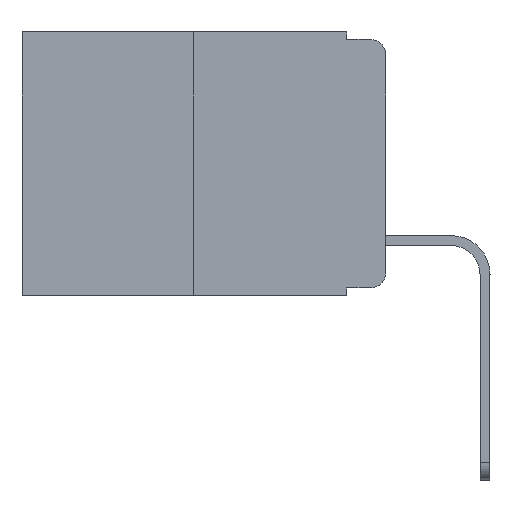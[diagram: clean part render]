
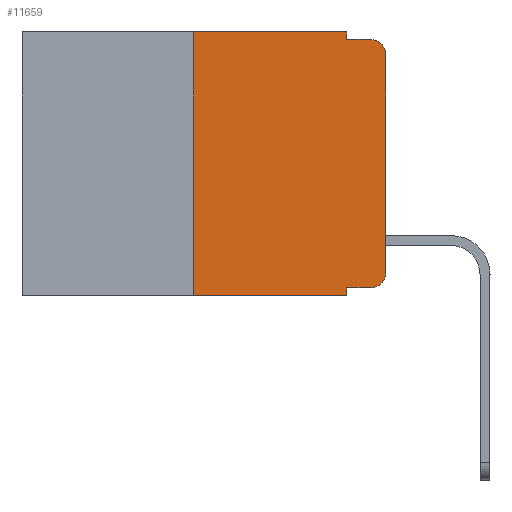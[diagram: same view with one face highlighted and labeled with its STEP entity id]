
A CAD part, left-side view. The second image highlights one B-rep face of the part: STEP entity #11659.
In plain terms, the highlighted planar face has unit normal (-1, 0, 0).
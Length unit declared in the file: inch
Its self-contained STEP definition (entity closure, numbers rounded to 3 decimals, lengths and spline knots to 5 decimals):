
#496 = DIRECTION ( 'NONE',  ( 1., 0., 0. ) ) ;
#709 = EDGE_LOOP ( 'NONE', ( #11144, #2116, #13449, #13961, #7534, #15008, #7653, #3943, #11089, #6713 ) ) ;
#839 = EDGE_CURVE ( 'NONE', #9653, #6945, #1702, .T. ) ;
#901 = EDGE_CURVE ( 'NONE', #14764, #1502, #4302, .T. ) ;
#1094 = CARTESIAN_POINT ( 'NONE',  ( 0., 0., 0. ) ) ;
#1298 = CARTESIAN_POINT ( 'NONE',  ( 0., 0.02, -0.333 ) ) ;
#1502 = VERTEX_POINT ( 'NONE', #8066 ) ;
#1522 = CARTESIAN_POINT ( 'NONE',  ( 0., 0.051, -0.01 ) ) ;
#1702 = CIRCLE ( 'NONE', #11332, 0.02 ) ;
#1748 = CARTESIAN_POINT ( 'NONE',  ( 0., 0.25, -0.343 ) ) ;
#1807 = CIRCLE ( 'NONE', #9581, 0.02 ) ;
#2116 = ORIENTED_EDGE ( 'NONE', *, *, #839, .T. ) ;
#2292 = VECTOR ( 'NONE', #12016, 39.37008 ) ;
#2937 = VERTEX_POINT ( 'NONE', #1298 ) ;
#3017 = DIRECTION ( 'NONE',  ( 0., -1., 0. ) ) ;
#3108 = CARTESIAN_POINT ( 'NONE',  ( 0., 0.473, 0. ) ) ;
#3184 = LINE ( 'NONE', #3108, #8839 ) ;
#3336 = DIRECTION ( 'NONE',  ( 0., 0., -1. ) ) ;
#3429 = CARTESIAN_POINT ( 'NONE',  ( 0., 0.051, 0. ) ) ;
#3559 = EDGE_CURVE ( 'NONE', #8387, #2937, #8196, .T. ) ;
#3943 = ORIENTED_EDGE ( 'NONE', *, *, #6161, .F. ) ;
#3948 = CARTESIAN_POINT ( 'NONE',  ( 0., 0.25, 0. ) ) ;
#4044 = CARTESIAN_POINT ( 'NONE',  ( 0., 0.051, -0.333 ) ) ;
#4079 = PLANE ( 'NONE',  #4419 ) ;
#4130 = DIRECTION ( 'NONE',  ( 0., 0., -1. ) ) ;
#4302 = LINE ( 'NONE', #6853, #14063 ) ;
#4419 = AXIS2_PLACEMENT_3D ( 'NONE', #7736, #496, #4130 ) ;
#4475 = DIRECTION ( 'NONE',  ( 0., -1., 0. ) ) ;
#4555 = CARTESIAN_POINT ( 'NONE',  ( 0., 0.25, 0. ) ) ;
#5433 = LINE ( 'NONE', #8692, #8498 ) ;
#5662 = LINE ( 'NONE', #1522, #7557 ) ;
#5698 = EDGE_CURVE ( 'NONE', #9456, #6945, #5662, .T. ) ;
#5762 = EDGE_CURVE ( 'NONE', #14777, #9653, #15029, .T. ) ;
#6000 = CARTESIAN_POINT ( 'NONE',  ( 0., 0.051, 0. ) ) ;
#6161 = EDGE_CURVE ( 'NONE', #8387, #1502, #9674, .T. ) ;
#6273 = FACE_OUTER_BOUND ( 'NONE', #709, .T. ) ;
#6713 = ORIENTED_EDGE ( 'NONE', *, *, #11077, .T. ) ;
#6776 = CARTESIAN_POINT ( 'NONE',  ( 0., 0.02, -0.313 ) ) ;
#6831 = CARTESIAN_POINT ( 'NONE',  ( 0., 0.051, -0.333 ) ) ;
#6853 = CARTESIAN_POINT ( 'NONE',  ( 0., 0.473, -0.343 ) ) ;
#6945 = VERTEX_POINT ( 'NONE', #12010 ) ;
#7286 = DIRECTION ( 'NONE',  ( 0., 0., -1. ) ) ;
#7534 = ORIENTED_EDGE ( 'NONE', *, *, #8431, .F. ) ;
#7557 = VECTOR ( 'NONE', #8630, 39.37008 ) ;
#7653 = ORIENTED_EDGE ( 'NONE', *, *, #901, .T. ) ;
#7736 = CARTESIAN_POINT ( 'NONE',  ( 0., 0.473, 0. ) ) ;
#8062 = VECTOR ( 'NONE', #9915, 39.37008 ) ;
#8066 = CARTESIAN_POINT ( 'NONE',  ( 0., 0.051, -0.343 ) ) ;
#8078 = CARTESIAN_POINT ( 'NONE',  ( 0., 0., -0.03 ) ) ;
#8196 = LINE ( 'NONE', #6831, #8738 ) ;
#8387 = VERTEX_POINT ( 'NONE', #4044 ) ;
#8431 = EDGE_CURVE ( 'NONE', #10648, #10008, #3184, .T. ) ;
#8498 = VECTOR ( 'NONE', #11091, 39.37008 ) ;
#8630 = DIRECTION ( 'NONE',  ( 0., -1., 0. ) ) ;
#8692 = CARTESIAN_POINT ( 'NONE',  ( 0., 0.051, 0. ) ) ;
#8738 = VECTOR ( 'NONE', #10573, 39.37008 ) ;
#8839 = VECTOR ( 'NONE', #3017, 39.37008 ) ;
#9292 = CARTESIAN_POINT ( 'NONE',  ( 0., 0.02, -0.03 ) ) ;
#9434 = DIRECTION ( 'NONE',  ( -1., 0., 0. ) ) ;
#9456 = VERTEX_POINT ( 'NONE', #10021 ) ;
#9581 = AXIS2_PLACEMENT_3D ( 'NONE', #6776, #12762, #10415 ) ;
#9653 = VERTEX_POINT ( 'NONE', #8078 ) ;
#9674 = LINE ( 'NONE', #6000, #15441 ) ;
#9915 = DIRECTION ( 'NONE',  ( 0., 0., 1. ) ) ;
#10008 = VERTEX_POINT ( 'NONE', #3429 ) ;
#10021 = CARTESIAN_POINT ( 'NONE',  ( 0., 0.051, -0.01 ) ) ;
#10315 = EDGE_CURVE ( 'NONE', #14764, #10648, #14759, .T. ) ;
#10415 = DIRECTION ( 'NONE',  ( 0., 0., -1. ) ) ;
#10573 = DIRECTION ( 'NONE',  ( 0., -1., 0. ) ) ;
#10648 = VERTEX_POINT ( 'NONE', #4555 ) ;
#11077 = EDGE_CURVE ( 'NONE', #2937, #14777, #1807, .T. ) ;
#11089 = ORIENTED_EDGE ( 'NONE', *, *, #3559, .T. ) ;
#11091 = DIRECTION ( 'NONE',  ( 0., 0., -1. ) ) ;
#11144 = ORIENTED_EDGE ( 'NONE', *, *, #5762, .T. ) ;
#11332 = AXIS2_PLACEMENT_3D ( 'NONE', #9292, #9434, #3336 ) ;
#11441 = CARTESIAN_POINT ( 'NONE',  ( 0., 0., -0.313 ) ) ;
#11659 = ADVANCED_FACE ( 'NONE', ( #6273 ), #4079, .F. ) ;
#12010 = CARTESIAN_POINT ( 'NONE',  ( 0., 0.02, -0.01 ) ) ;
#12016 = DIRECTION ( 'NONE',  ( 0., 0., 1. ) ) ;
#12762 = DIRECTION ( 'NONE',  ( -1., 0., 0. ) ) ;
#13449 = ORIENTED_EDGE ( 'NONE', *, *, #5698, .F. ) ;
#13961 = ORIENTED_EDGE ( 'NONE', *, *, #14683, .F. ) ;
#14063 = VECTOR ( 'NONE', #4475, 39.37008 ) ;
#14683 = EDGE_CURVE ( 'NONE', #10008, #9456, #5433, .T. ) ;
#14759 = LINE ( 'NONE', #3948, #8062 ) ;
#14764 = VERTEX_POINT ( 'NONE', #1748 ) ;
#14777 = VERTEX_POINT ( 'NONE', #11441 ) ;
#15008 = ORIENTED_EDGE ( 'NONE', *, *, #10315, .F. ) ;
#15029 = LINE ( 'NONE', #1094, #2292 ) ;
#15441 = VECTOR ( 'NONE', #7286, 39.37008 ) ;
